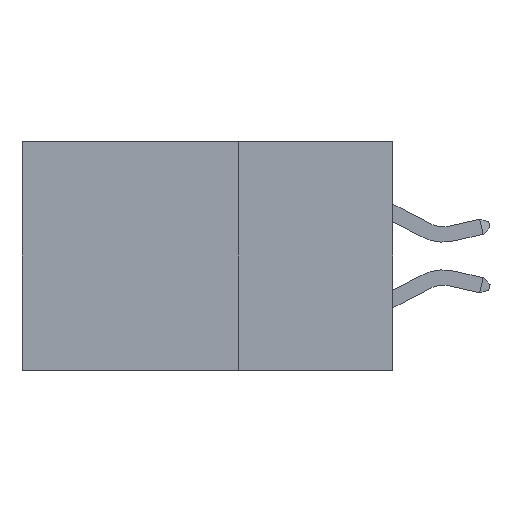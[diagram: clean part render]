
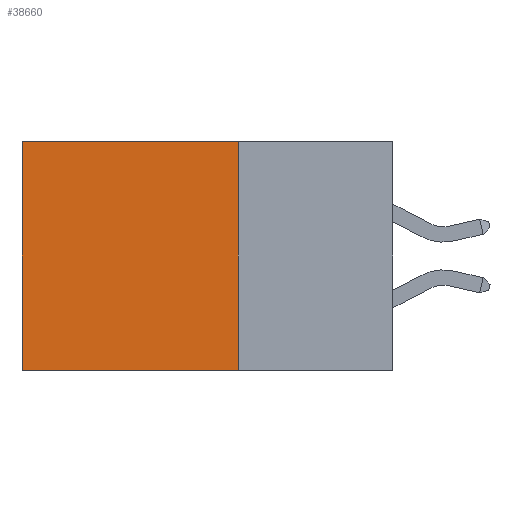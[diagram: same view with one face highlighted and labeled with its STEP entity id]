
A CAD part, left-side view. The second image highlights one B-rep face of the part: STEP entity #38660.
In plain terms, the highlighted planar face has unit normal (-1, 0, 0).
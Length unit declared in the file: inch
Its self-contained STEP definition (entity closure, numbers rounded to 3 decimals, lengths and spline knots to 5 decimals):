
#1300 = EDGE_CURVE ( 'NONE', #10101, #32285, #11712, .T. ) ;
#1323 = VECTOR ( 'NONE', #16087, 39.37008 ) ;
#2001 = VERTEX_POINT ( 'NONE', #4133 ) ;
#2502 = EDGE_CURVE ( 'NONE', #8498, #2001, #24852, .T. ) ;
#3692 = EDGE_CURVE ( 'NONE', #10101, #8498, #20990, .T. ) ;
#3848 = DIRECTION ( 'NONE',  ( 0., 0., -1. ) ) ;
#4133 = CARTESIAN_POINT ( 'NONE',  ( 0.2875, 0.6, -0.37 ) ) ;
#6153 = VECTOR ( 'NONE', #9503, 39.37008 ) ;
#8498 = VERTEX_POINT ( 'NONE', #43243 ) ;
#9263 = CARTESIAN_POINT ( 'NONE',  ( 0.2875, 0.25, 0. ) ) ;
#9503 = DIRECTION ( 'NONE',  ( 0., 1., 0. ) ) ;
#10101 = VERTEX_POINT ( 'NONE', #37809 ) ;
#10117 = VECTOR ( 'NONE', #37279, 39.37008 ) ;
#11712 = LINE ( 'NONE', #20698, #10117 ) ;
#13927 = AXIS2_PLACEMENT_3D ( 'NONE', #17114, #17561, #41002 ) ;
#14694 = LINE ( 'NONE', #28120, #26949 ) ;
#16087 = DIRECTION ( 'NONE',  ( 0., 0., -1. ) ) ;
#17114 = CARTESIAN_POINT ( 'NONE',  ( 0.2875, 0.25, 0. ) ) ;
#17561 = DIRECTION ( 'NONE',  ( 1., 0., 0. ) ) ;
#18412 = EDGE_LOOP ( 'NONE', ( #33304, #22195, #37020, #24144 ) ) ;
#20393 = EDGE_CURVE ( 'NONE', #32285, #2001, #14694, .T. ) ;
#20698 = CARTESIAN_POINT ( 'NONE',  ( 0.2875, 0.25, 0. ) ) ;
#20990 = LINE ( 'NONE', #9263, #1323 ) ;
#21996 = CARTESIAN_POINT ( 'NONE',  ( 0.2875, 0.6, 0. ) ) ;
#22195 = ORIENTED_EDGE ( 'NONE', *, *, #2502, .F. ) ;
#24144 = ORIENTED_EDGE ( 'NONE', *, *, #1300, .T. ) ;
#24852 = LINE ( 'NONE', #36464, #6153 ) ;
#26949 = VECTOR ( 'NONE', #3848, 39.37008 ) ;
#28120 = CARTESIAN_POINT ( 'NONE',  ( 0.2875, 0.6, 0. ) ) ;
#32285 = VERTEX_POINT ( 'NONE', #21996 ) ;
#33304 = ORIENTED_EDGE ( 'NONE', *, *, #20393, .T. ) ;
#34124 = PLANE ( 'NONE',  #13927 ) ;
#36464 = CARTESIAN_POINT ( 'NONE',  ( 0.2875, 0.25, -0.37 ) ) ;
#37020 = ORIENTED_EDGE ( 'NONE', *, *, #3692, .F. ) ;
#37279 = DIRECTION ( 'NONE',  ( 0., 1., 0. ) ) ;
#37809 = CARTESIAN_POINT ( 'NONE',  ( 0.2875, 0.25, 0. ) ) ;
#38660 = ADVANCED_FACE ( 'NONE', ( #39381 ), #34124, .F. ) ;
#39381 = FACE_OUTER_BOUND ( 'NONE', #18412, .T. ) ;
#41002 = DIRECTION ( 'NONE',  ( 0., 0., -1. ) ) ;
#43243 = CARTESIAN_POINT ( 'NONE',  ( 0.2875, 0.25, -0.37 ) ) ;
